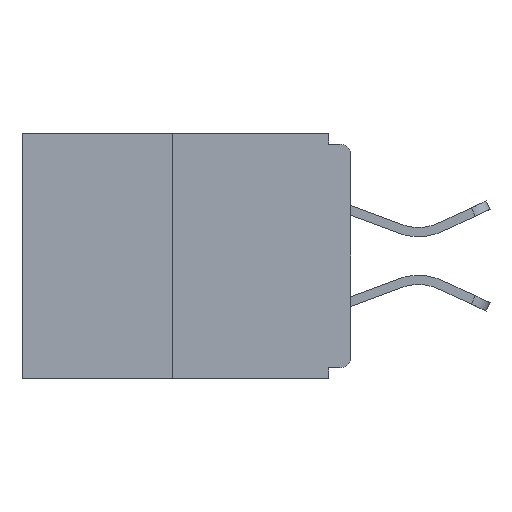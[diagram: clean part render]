
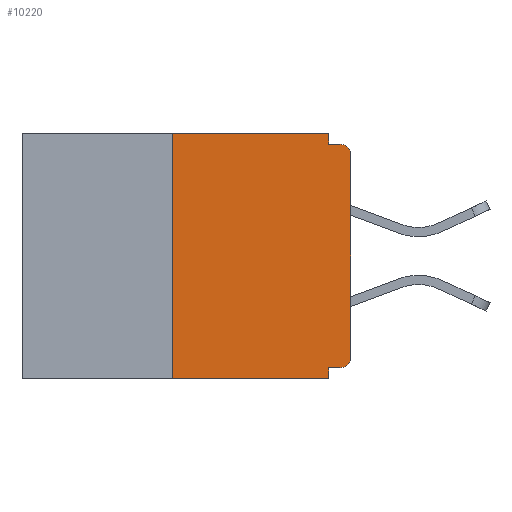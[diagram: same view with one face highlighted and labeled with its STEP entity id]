
A CAD part, left-side view. The second image highlights one B-rep face of the part: STEP entity #10220.
In plain terms, the highlighted planar face has unit normal (-1, 0, 0).
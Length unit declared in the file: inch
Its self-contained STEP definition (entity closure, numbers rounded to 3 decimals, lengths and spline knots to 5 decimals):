
#24 = VECTOR ( 'NONE', #15054, 39.37008 ) ;
#898 = AXIS2_PLACEMENT_3D ( 'NONE', #23543, #12004, #2601 ) ;
#1221 = VECTOR ( 'NONE', #16562, 39.37008 ) ;
#1315 = CARTESIAN_POINT ( 'NONE',  ( 0., 0., -0.313 ) ) ;
#1324 = ORIENTED_EDGE ( 'NONE', *, *, #7339, .T. ) ;
#1335 = EDGE_CURVE ( 'NONE', #1403, #5723, #6364, .T. ) ;
#1403 = VERTEX_POINT ( 'NONE', #18364 ) ;
#2015 = CARTESIAN_POINT ( 'NONE',  ( 0., 0.031, 0. ) ) ;
#2569 = DIRECTION ( 'NONE',  ( 0., 0., 1. ) ) ;
#2601 = DIRECTION ( 'NONE',  ( 0., 0., -1. ) ) ;
#2768 = DIRECTION ( 'NONE',  ( 0., -1., 0. ) ) ;
#2972 = CARTESIAN_POINT ( 'NONE',  ( 0., 0., -0.328 ) ) ;
#3490 = CARTESIAN_POINT ( 'NONE',  ( 0., 0.46, 0. ) ) ;
#3588 = VECTOR ( 'NONE', #4052, 39.37008 ) ;
#3961 = AXIS2_PLACEMENT_3D ( 'NONE', #10147, #12092, #11765 ) ;
#4052 = DIRECTION ( 'NONE',  ( 0., 0., -1. ) ) ;
#4653 = CARTESIAN_POINT ( 'NONE',  ( 0., 0.015, -0.015 ) ) ;
#4704 = ORIENTED_EDGE ( 'NONE', *, *, #11377, .T. ) ;
#4858 = VERTEX_POINT ( 'NONE', #7704 ) ;
#5723 = VERTEX_POINT ( 'NONE', #18665 ) ;
#5899 = DIRECTION ( 'NONE',  ( 0., -1., 0. ) ) ;
#6080 = DIRECTION ( 'NONE',  ( 1., 0., 0. ) ) ;
#6364 = LINE ( 'NONE', #3490, #1221 ) ;
#6678 = ORIENTED_EDGE ( 'NONE', *, *, #21543, .F. ) ;
#6852 = VERTEX_POINT ( 'NONE', #8749 ) ;
#7190 = EDGE_CURVE ( 'NONE', #17349, #6852, #19500, .T. ) ;
#7339 = EDGE_CURVE ( 'NONE', #15137, #8592, #14358, .T. ) ;
#7704 = CARTESIAN_POINT ( 'NONE',  ( 0., 0.25, -0.343 ) ) ;
#7734 = EDGE_LOOP ( 'NONE', ( #13474, #24168, #4704, #16443, #6678, #23481, #9287, #1324, #19461, #17985 ) ) ;
#7915 = CARTESIAN_POINT ( 'NONE',  ( 0., 0., -0.015 ) ) ;
#8074 = VERTEX_POINT ( 'NONE', #22322 ) ;
#8191 = PLANE ( 'NONE',  #10462 ) ;
#8435 = CARTESIAN_POINT ( 'NONE',  ( 0., 0.46, -0.343 ) ) ;
#8556 = DIRECTION ( 'NONE',  ( 0., 1., 0. ) ) ;
#8592 = VERTEX_POINT ( 'NONE', #4653 ) ;
#8749 = CARTESIAN_POINT ( 'NONE',  ( 0., 0.031, -0.343 ) ) ;
#9200 = VECTOR ( 'NONE', #13878, 39.37008 ) ;
#9287 = ORIENTED_EDGE ( 'NONE', *, *, #18016, .T. ) ;
#9790 = EDGE_CURVE ( 'NONE', #4858, #1403, #12104, .T. ) ;
#10147 = CARTESIAN_POINT ( 'NONE',  ( 0., 0.015, -0.313 ) ) ;
#10220 = ADVANCED_FACE ( 'NONE', ( #23521 ), #8191, .F. ) ;
#10275 = EDGE_CURVE ( 'NONE', #5723, #8074, #15105, .T. ) ;
#10462 = AXIS2_PLACEMENT_3D ( 'NONE', #15882, #6080, #13791 ) ;
#11377 = EDGE_CURVE ( 'NONE', #4858, #6852, #11696, .T. ) ;
#11696 = LINE ( 'NONE', #8435, #22265 ) ;
#11765 = DIRECTION ( 'NONE',  ( 0., 0., -1. ) ) ;
#11920 = CARTESIAN_POINT ( 'NONE',  ( 0., 0.031, -0.343 ) ) ;
#11999 = VECTOR ( 'NONE', #5899, 39.37008 ) ;
#12004 = DIRECTION ( 'NONE',  ( -1., 0., 0. ) ) ;
#12092 = DIRECTION ( 'NONE',  ( -1., 0., 0. ) ) ;
#12104 = LINE ( 'NONE', #18105, #21455 ) ;
#13474 = ORIENTED_EDGE ( 'NONE', *, *, #1335, .F. ) ;
#13791 = DIRECTION ( 'NONE',  ( 0., 0., -1. ) ) ;
#13832 = LINE ( 'NONE', #7915, #11999 ) ;
#13878 = DIRECTION ( 'NONE',  ( 0., 0., -1. ) ) ;
#13975 = CARTESIAN_POINT ( 'NONE',  ( 0., 0., 0. ) ) ;
#14240 = LINE ( 'NONE', #2972, #14835 ) ;
#14329 = EDGE_CURVE ( 'NONE', #8074, #8592, #13832, .T. ) ;
#14358 = CIRCLE ( 'NONE', #898, 0.015 ) ;
#14835 = VECTOR ( 'NONE', #8556, 39.37008 ) ;
#15054 = DIRECTION ( 'NONE',  ( 0., 0., 1. ) ) ;
#15085 = CARTESIAN_POINT ( 'NONE',  ( 0., 0.015, -0.328 ) ) ;
#15105 = LINE ( 'NONE', #2015, #3588 ) ;
#15137 = VERTEX_POINT ( 'NONE', #23906 ) ;
#15882 = CARTESIAN_POINT ( 'NONE',  ( 0., 0.46, 0. ) ) ;
#16443 = ORIENTED_EDGE ( 'NONE', *, *, #7190, .F. ) ;
#16562 = DIRECTION ( 'NONE',  ( 0., -1., 0. ) ) ;
#17228 = LINE ( 'NONE', #13975, #24 ) ;
#17277 = CIRCLE ( 'NONE', #3961, 0.015 ) ;
#17349 = VERTEX_POINT ( 'NONE', #23322 ) ;
#17591 = VERTEX_POINT ( 'NONE', #1315 ) ;
#17985 = ORIENTED_EDGE ( 'NONE', *, *, #10275, .F. ) ;
#18016 = EDGE_CURVE ( 'NONE', #17591, #15137, #17228, .T. ) ;
#18105 = CARTESIAN_POINT ( 'NONE',  ( 0., 0.25, 0. ) ) ;
#18364 = CARTESIAN_POINT ( 'NONE',  ( 0., 0.25, 0. ) ) ;
#18665 = CARTESIAN_POINT ( 'NONE',  ( 0., 0.031, 0. ) ) ;
#19461 = ORIENTED_EDGE ( 'NONE', *, *, #14329, .F. ) ;
#19500 = LINE ( 'NONE', #11920, #9200 ) ;
#20518 = VERTEX_POINT ( 'NONE', #15085 ) ;
#20743 = EDGE_CURVE ( 'NONE', #20518, #17591, #17277, .T. ) ;
#21455 = VECTOR ( 'NONE', #2569, 39.37008 ) ;
#21543 = EDGE_CURVE ( 'NONE', #20518, #17349, #14240, .T. ) ;
#22265 = VECTOR ( 'NONE', #2768, 39.37008 ) ;
#22322 = CARTESIAN_POINT ( 'NONE',  ( 0., 0.031, -0.015 ) ) ;
#23322 = CARTESIAN_POINT ( 'NONE',  ( 0., 0.031, -0.328 ) ) ;
#23481 = ORIENTED_EDGE ( 'NONE', *, *, #20743, .T. ) ;
#23521 = FACE_OUTER_BOUND ( 'NONE', #7734, .T. ) ;
#23543 = CARTESIAN_POINT ( 'NONE',  ( 0., 0.015, -0.03 ) ) ;
#23906 = CARTESIAN_POINT ( 'NONE',  ( 0., 0., -0.03 ) ) ;
#24168 = ORIENTED_EDGE ( 'NONE', *, *, #9790, .F. ) ;
